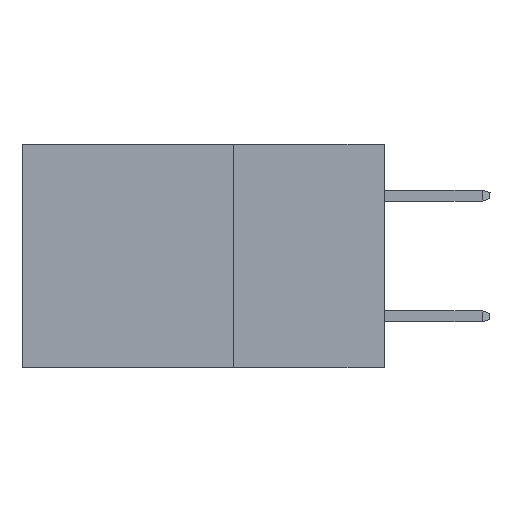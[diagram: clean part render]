
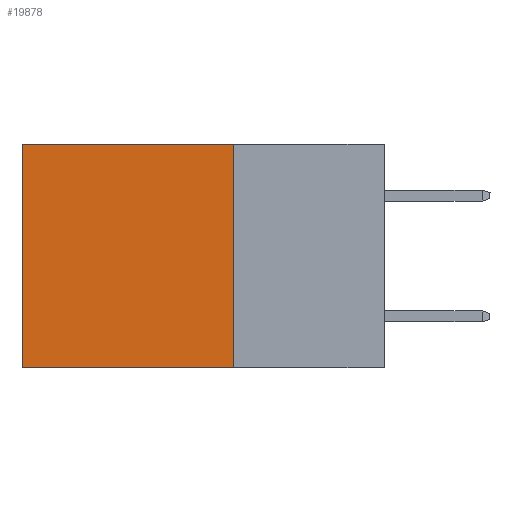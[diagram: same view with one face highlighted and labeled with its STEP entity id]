
A CAD part, left-side view. The second image highlights one B-rep face of the part: STEP entity #19878.
In plain terms, the highlighted planar face has unit normal (-1, 0, 0).
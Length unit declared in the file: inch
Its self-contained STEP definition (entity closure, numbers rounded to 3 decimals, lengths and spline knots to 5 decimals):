
#143 = EDGE_CURVE ( 'NONE', #13974, #2044, #14564, .T. ) ;
#591 = VECTOR ( 'NONE', #18230, 39.37008 ) ;
#1739 = ORIENTED_EDGE ( 'NONE', *, *, #11534, .F. ) ;
#1974 = CARTESIAN_POINT ( 'NONE',  ( 0.298, 0.25, -0.37 ) ) ;
#2044 = VERTEX_POINT ( 'NONE', #1974 ) ;
#3299 = DIRECTION ( 'NONE',  ( 1., 0., 0. ) ) ;
#5086 = DIRECTION ( 'NONE',  ( 0., 1., 0. ) ) ;
#6660 = ORIENTED_EDGE ( 'NONE', *, *, #19515, .T. ) ;
#6842 = PLANE ( 'NONE',  #21227 ) ;
#8152 = VECTOR ( 'NONE', #11694, 39.37008 ) ;
#8522 = CARTESIAN_POINT ( 'NONE',  ( 0.298, 0.25, 0. ) ) ;
#10189 = VERTEX_POINT ( 'NONE', #15721 ) ;
#11075 = LINE ( 'NONE', #20254, #591 ) ;
#11193 = ORIENTED_EDGE ( 'NONE', *, *, #13794, .T. ) ;
#11518 = LINE ( 'NONE', #22629, #19886 ) ;
#11534 = EDGE_CURVE ( 'NONE', #2044, #16982, #11075, .T. ) ;
#11694 = DIRECTION ( 'NONE',  ( 0., 0., -1. ) ) ;
#13645 = DIRECTION ( 'NONE',  ( 0., 0., -1. ) ) ;
#13745 = CARTESIAN_POINT ( 'NONE',  ( 0.298, 0.25, 0. ) ) ;
#13794 = EDGE_CURVE ( 'NONE', #10189, #16982, #11518, .T. ) ;
#13974 = VERTEX_POINT ( 'NONE', #19062 ) ;
#14262 = CARTESIAN_POINT ( 'NONE',  ( 0.298, 0.6, -0.37 ) ) ;
#14564 = LINE ( 'NONE', #8522, #8152 ) ;
#14717 = LINE ( 'NONE', #13745, #21982 ) ;
#15586 = CARTESIAN_POINT ( 'NONE',  ( 0.298, 0.25, 0. ) ) ;
#15721 = CARTESIAN_POINT ( 'NONE',  ( 0.298, 0.6, 0. ) ) ;
#16982 = VERTEX_POINT ( 'NONE', #14262 ) ;
#17795 = EDGE_LOOP ( 'NONE', ( #11193, #1739, #19957, #6660 ) ) ;
#18230 = DIRECTION ( 'NONE',  ( 0., 1., 0. ) ) ;
#19062 = CARTESIAN_POINT ( 'NONE',  ( 0.298, 0.25, 0. ) ) ;
#19171 = FACE_OUTER_BOUND ( 'NONE', #17795, .T. ) ;
#19515 = EDGE_CURVE ( 'NONE', #13974, #10189, #14717, .T. ) ;
#19878 = ADVANCED_FACE ( 'NONE', ( #19171 ), #6842, .F. ) ;
#19886 = VECTOR ( 'NONE', #13645, 39.37008 ) ;
#19957 = ORIENTED_EDGE ( 'NONE', *, *, #143, .F. ) ;
#20254 = CARTESIAN_POINT ( 'NONE',  ( 0.298, 0.25, -0.37 ) ) ;
#21227 = AXIS2_PLACEMENT_3D ( 'NONE', #15586, #3299, #22703 ) ;
#21982 = VECTOR ( 'NONE', #5086, 39.37008 ) ;
#22629 = CARTESIAN_POINT ( 'NONE',  ( 0.298, 0.6, 0. ) ) ;
#22703 = DIRECTION ( 'NONE',  ( 0., 0., -1. ) ) ;
